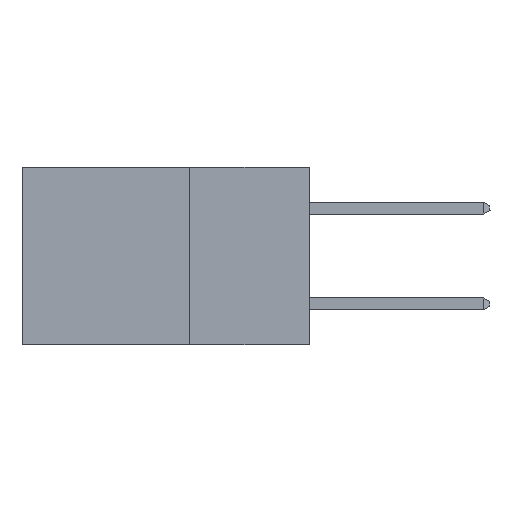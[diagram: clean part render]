
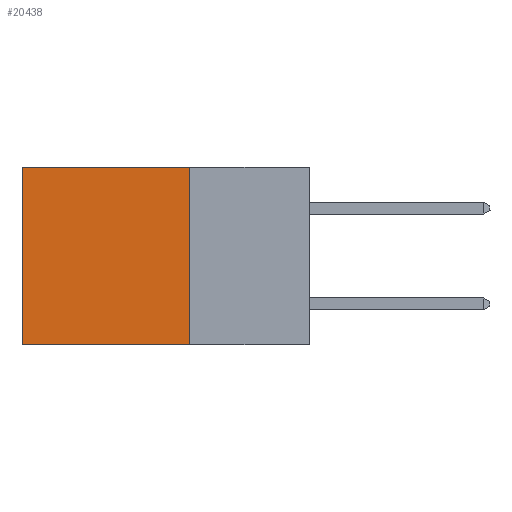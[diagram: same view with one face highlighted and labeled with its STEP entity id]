
A CAD part, left-side view. The second image highlights one B-rep face of the part: STEP entity #20438.
In plain terms, the highlighted planar face has unit normal (-1, 0, 0).
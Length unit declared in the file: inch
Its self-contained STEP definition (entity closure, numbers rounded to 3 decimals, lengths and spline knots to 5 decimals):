
#312 = EDGE_CURVE ( 'NONE', #12435, #2196, #14566, .T. ) ;
#523 = ORIENTED_EDGE ( 'NONE', *, *, #17825, .T. ) ;
#1893 = LINE ( 'NONE', #11493, #20172 ) ;
#1957 = CARTESIAN_POINT ( 'NONE',  ( 0.2875, 0.25, 0. ) ) ;
#2029 = DIRECTION ( 'NONE',  ( 0., 0., -1. ) ) ;
#2196 = VERTEX_POINT ( 'NONE', #21016 ) ;
#2304 = AXIS2_PLACEMENT_3D ( 'NONE', #1957, #14343, #2029 ) ;
#3128 = LINE ( 'NONE', #3586, #21100 ) ;
#3422 = EDGE_CURVE ( 'NONE', #12435, #20002, #3128, .T. ) ;
#3586 = CARTESIAN_POINT ( 'NONE',  ( 0.2875, 0.25, 0. ) ) ;
#4277 = DIRECTION ( 'NONE',  ( 0., 0., -1. ) ) ;
#6223 = ORIENTED_EDGE ( 'NONE', *, *, #16348, .F. ) ;
#8205 = DIRECTION ( 'NONE',  ( 0., 0., -1. ) ) ;
#8820 = ORIENTED_EDGE ( 'NONE', *, *, #3422, .T. ) ;
#9819 = VECTOR ( 'NONE', #22255, 39.37008 ) ;
#9944 = FACE_OUTER_BOUND ( 'NONE', #20691, .T. ) ;
#11493 = CARTESIAN_POINT ( 'NONE',  ( 0.2875, 0.6, 0. ) ) ;
#12435 = VERTEX_POINT ( 'NONE', #16129 ) ;
#14031 = VECTOR ( 'NONE', #4277, 39.37008 ) ;
#14326 = VERTEX_POINT ( 'NONE', #16729 ) ;
#14343 = DIRECTION ( 'NONE',  ( 1., 0., 0. ) ) ;
#14566 = LINE ( 'NONE', #16947, #14031 ) ;
#14886 = CARTESIAN_POINT ( 'NONE',  ( 0.2875, 0.6, 0. ) ) ;
#16129 = CARTESIAN_POINT ( 'NONE',  ( 0.2875, 0.25, 0. ) ) ;
#16348 = EDGE_CURVE ( 'NONE', #2196, #14326, #18237, .T. ) ;
#16729 = CARTESIAN_POINT ( 'NONE',  ( 0.2875, 0.6, -0.37 ) ) ;
#16947 = CARTESIAN_POINT ( 'NONE',  ( 0.2875, 0.25, 0. ) ) ;
#17825 = EDGE_CURVE ( 'NONE', #20002, #14326, #1893, .T. ) ;
#18237 = LINE ( 'NONE', #22404, #9819 ) ;
#20002 = VERTEX_POINT ( 'NONE', #14886 ) ;
#20172 = VECTOR ( 'NONE', #8205, 39.37008 ) ;
#20438 = ADVANCED_FACE ( 'NONE', ( #9944 ), #22383, .F. ) ;
#20691 = EDGE_LOOP ( 'NONE', ( #523, #6223, #20858, #8820 ) ) ;
#20858 = ORIENTED_EDGE ( 'NONE', *, *, #312, .F. ) ;
#21016 = CARTESIAN_POINT ( 'NONE',  ( 0.2875, 0.25, -0.37 ) ) ;
#21100 = VECTOR ( 'NONE', #21323, 39.37008 ) ;
#21323 = DIRECTION ( 'NONE',  ( 0., 1., 0. ) ) ;
#22255 = DIRECTION ( 'NONE',  ( 0., 1., 0. ) ) ;
#22383 = PLANE ( 'NONE',  #2304 ) ;
#22404 = CARTESIAN_POINT ( 'NONE',  ( 0.2875, 0.25, -0.37 ) ) ;
